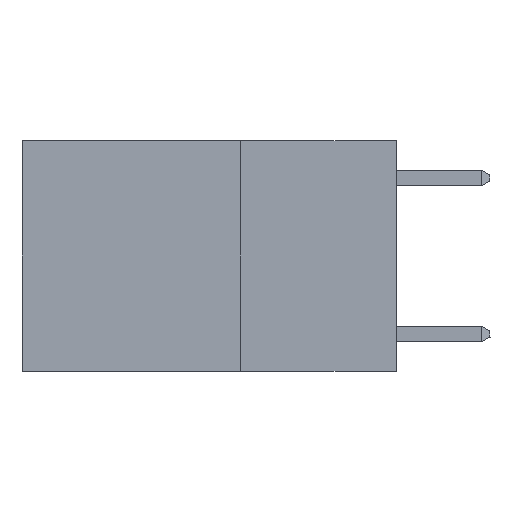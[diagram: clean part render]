
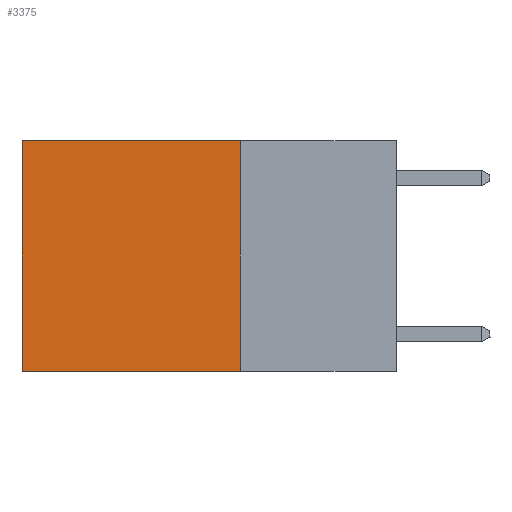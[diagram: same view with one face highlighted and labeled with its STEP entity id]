
A CAD part, left-side view. The second image highlights one B-rep face of the part: STEP entity #3375.
In plain terms, the highlighted planar face has unit normal (-1, 0, 0).
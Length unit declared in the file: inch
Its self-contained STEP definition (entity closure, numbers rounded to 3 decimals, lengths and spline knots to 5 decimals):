
#1595 = VERTEX_POINT ( 'NONE', #3031 ) ;
#2210 = DIRECTION ( 'NONE',  ( 0., 0., -1. ) ) ;
#2215 = ORIENTED_EDGE ( 'NONE', *, *, #10246, .F. ) ;
#2290 = VECTOR ( 'NONE', #2210, 39.37008 ) ;
#2663 = CARTESIAN_POINT ( 'NONE',  ( 0.2625, 0.25, 0. ) ) ;
#2781 = DIRECTION ( 'NONE',  ( 0., 1., 0. ) ) ;
#3031 = CARTESIAN_POINT ( 'NONE',  ( 0.2625, 0.25, 0. ) ) ;
#3375 = ADVANCED_FACE ( 'NONE', ( #9159 ), #12630, .F. ) ;
#3999 = DIRECTION ( 'NONE',  ( 1., 0., 0. ) ) ;
#5115 = CARTESIAN_POINT ( 'NONE',  ( 0.2625, 0.6, 0. ) ) ;
#5469 = ORIENTED_EDGE ( 'NONE', *, *, #13318, .T. ) ;
#6404 = CARTESIAN_POINT ( 'NONE',  ( 0.2625, 0.6, 0. ) ) ;
#7578 = CARTESIAN_POINT ( 'NONE',  ( 0.2625, 0.25, -0.37 ) ) ;
#7932 = LINE ( 'NONE', #2663, #15066 ) ;
#8414 = CARTESIAN_POINT ( 'NONE',  ( 0.2625, 0.6, -0.37 ) ) ;
#9159 = FACE_OUTER_BOUND ( 'NONE', #14040, .T. ) ;
#10022 = LINE ( 'NONE', #5115, #2290 ) ;
#10246 = EDGE_CURVE ( 'NONE', #10868, #17483, #15130, .T. ) ;
#10323 = EDGE_CURVE ( 'NONE', #14057, #17483, #10022, .T. ) ;
#10770 = DIRECTION ( 'NONE',  ( 0., 1., 0. ) ) ;
#10868 = VERTEX_POINT ( 'NONE', #7578 ) ;
#11366 = DIRECTION ( 'NONE',  ( 0., 0., -1. ) ) ;
#12506 = ORIENTED_EDGE ( 'NONE', *, *, #13211, .F. ) ;
#12572 = CARTESIAN_POINT ( 'NONE',  ( 0.2625, 0.25, 0. ) ) ;
#12630 = PLANE ( 'NONE',  #13161 ) ;
#13161 = AXIS2_PLACEMENT_3D ( 'NONE', #12572, #3999, #14047 ) ;
#13211 = EDGE_CURVE ( 'NONE', #1595, #10868, #7932, .T. ) ;
#13318 = EDGE_CURVE ( 'NONE', #1595, #14057, #17917, .T. ) ;
#13737 = VECTOR ( 'NONE', #2781, 39.37008 ) ;
#14040 = EDGE_LOOP ( 'NONE', ( #17429, #2215, #12506, #5469 ) ) ;
#14047 = DIRECTION ( 'NONE',  ( 0., 0., -1. ) ) ;
#14057 = VERTEX_POINT ( 'NONE', #6404 ) ;
#14680 = VECTOR ( 'NONE', #10770, 39.37008 ) ;
#14857 = CARTESIAN_POINT ( 'NONE',  ( 0.2625, 0.25, 0. ) ) ;
#14984 = CARTESIAN_POINT ( 'NONE',  ( 0.2625, 0.25, -0.37 ) ) ;
#15066 = VECTOR ( 'NONE', #11366, 39.37008 ) ;
#15130 = LINE ( 'NONE', #14984, #14680 ) ;
#17429 = ORIENTED_EDGE ( 'NONE', *, *, #10323, .T. ) ;
#17483 = VERTEX_POINT ( 'NONE', #8414 ) ;
#17917 = LINE ( 'NONE', #14857, #13737 ) ;
